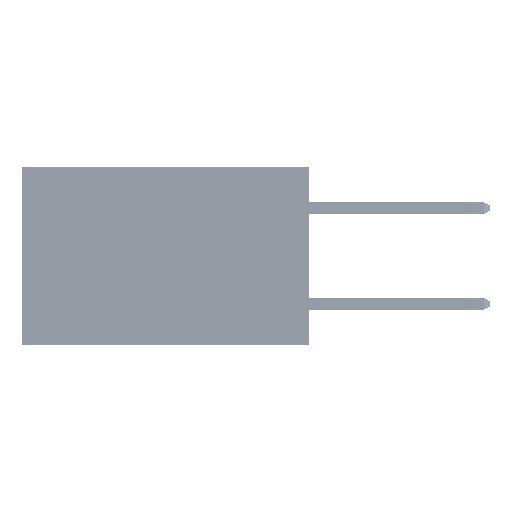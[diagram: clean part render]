
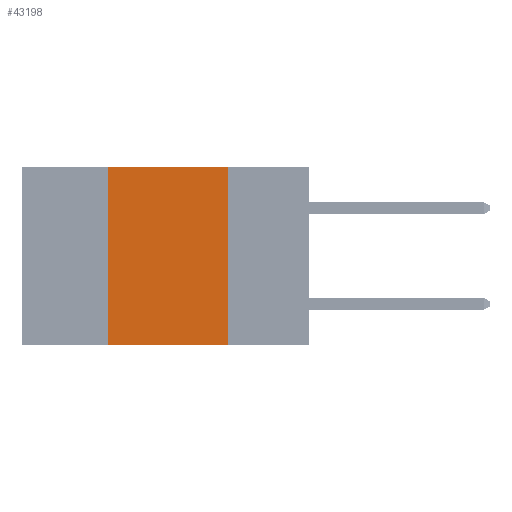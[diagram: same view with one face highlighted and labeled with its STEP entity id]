
A CAD part, left-side view. The second image highlights one B-rep face of the part: STEP entity #43198.
In plain terms, the highlighted planar face has unit normal (-1, 0, 0).
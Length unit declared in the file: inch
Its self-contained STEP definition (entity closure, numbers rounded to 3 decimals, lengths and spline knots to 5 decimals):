
#975 = ORIENTED_EDGE ( 'NONE', *, *, #8835, .F. ) ;
#2827 = FACE_OUTER_BOUND ( 'NONE', #45415, .T. ) ;
#3142 = LINE ( 'NONE', #14004, #18485 ) ;
#4931 = VERTEX_POINT ( 'NONE', #15370 ) ;
#5813 = DIRECTION ( 'NONE',  ( 0., -1., 0. ) ) ;
#6195 = VECTOR ( 'NONE', #34144, 39.37008 ) ;
#6450 = ORIENTED_EDGE ( 'NONE', *, *, #20148, .T. ) ;
#6576 = ORIENTED_EDGE ( 'NONE', *, *, #22752, .F. ) ;
#6617 = CARTESIAN_POINT ( 'NONE',  ( 0., 0.42, 0. ) ) ;
#7991 = CARTESIAN_POINT ( 'NONE',  ( 0., 0.42, 0. ) ) ;
#8835 = EDGE_CURVE ( 'NONE', #45477, #44462, #3142, .T. ) ;
#10588 = LINE ( 'NONE', #19923, #44690 ) ;
#12278 = CARTESIAN_POINT ( 'NONE',  ( 0., 0.17, -0.37 ) ) ;
#14004 = CARTESIAN_POINT ( 'NONE',  ( 0., 0.17, 0. ) ) ;
#15209 = LINE ( 'NONE', #31530, #43998 ) ;
#15370 = CARTESIAN_POINT ( 'NONE',  ( 0., 0.42, -0.37 ) ) ;
#16046 = DIRECTION ( 'NONE',  ( 0., 0., -1. ) ) ;
#18485 = VECTOR ( 'NONE', #43600, 39.37008 ) ;
#19923 = CARTESIAN_POINT ( 'NONE',  ( 0., 0.6, -0.37 ) ) ;
#20148 = EDGE_CURVE ( 'NONE', #4931, #44462, #10588, .T. ) ;
#22752 = EDGE_CURVE ( 'NONE', #4931, #46612, #26242, .T. ) ;
#22761 = PLANE ( 'NONE',  #33511 ) ;
#25516 = CARTESIAN_POINT ( 'NONE',  ( 0., 0.6, 0. ) ) ;
#25844 = CARTESIAN_POINT ( 'NONE',  ( 0., 0.17, 0. ) ) ;
#26242 = LINE ( 'NONE', #7991, #6195 ) ;
#31530 = CARTESIAN_POINT ( 'NONE',  ( 0., 0.6, 0. ) ) ;
#33493 = ORIENTED_EDGE ( 'NONE', *, *, #43276, .F. ) ;
#33511 = AXIS2_PLACEMENT_3D ( 'NONE', #25516, #34968, #16046 ) ;
#34144 = DIRECTION ( 'NONE',  ( 0., 0., 1. ) ) ;
#34968 = DIRECTION ( 'NONE',  ( 1., 0., 0. ) ) ;
#35092 = DIRECTION ( 'NONE',  ( 0., -1., 0. ) ) ;
#43198 = ADVANCED_FACE ( 'NONE', ( #2827 ), #22761, .F. ) ;
#43276 = EDGE_CURVE ( 'NONE', #46612, #45477, #15209, .T. ) ;
#43600 = DIRECTION ( 'NONE',  ( 0., 0., -1. ) ) ;
#43998 = VECTOR ( 'NONE', #5813, 39.37008 ) ;
#44462 = VERTEX_POINT ( 'NONE', #12278 ) ;
#44690 = VECTOR ( 'NONE', #35092, 39.37008 ) ;
#45415 = EDGE_LOOP ( 'NONE', ( #975, #33493, #6576, #6450 ) ) ;
#45477 = VERTEX_POINT ( 'NONE', #25844 ) ;
#46612 = VERTEX_POINT ( 'NONE', #6617 ) ;
